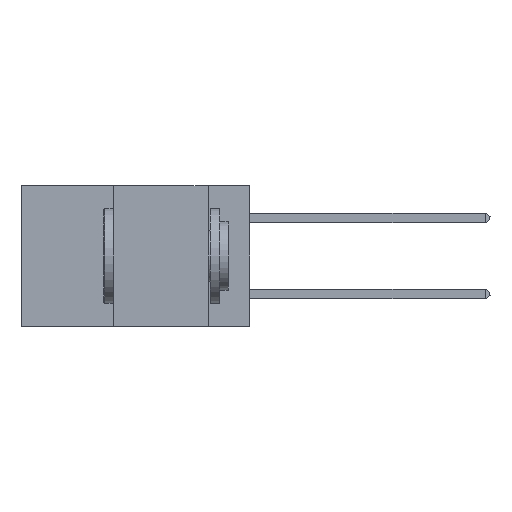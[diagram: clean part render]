
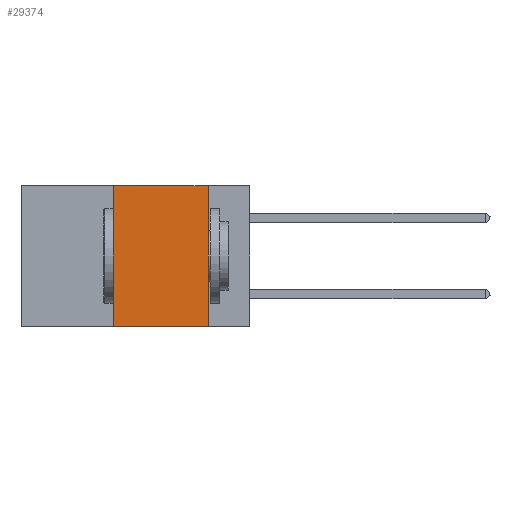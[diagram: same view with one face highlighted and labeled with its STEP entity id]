
A CAD part, left-side view. The second image highlights one B-rep face of the part: STEP entity #29374.
In plain terms, the highlighted planar face has unit normal (-1, 0, 0).
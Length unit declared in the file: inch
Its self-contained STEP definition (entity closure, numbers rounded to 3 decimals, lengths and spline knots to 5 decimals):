
#722 = EDGE_CURVE ( 'NONE', #38622, #37734, #21230, .T. ) ;
#1094 = EDGE_CURVE ( 'NONE', #31111, #38622, #18928, .T. ) ;
#1618 = VECTOR ( 'NONE', #26236, 39.37008 ) ;
#3147 = EDGE_CURVE ( 'NONE', #31111, #35357, #33803, .T. ) ;
#4628 = DIRECTION ( 'NONE',  ( 0., -1., 0. ) ) ;
#5275 = ORIENTED_EDGE ( 'NONE', *, *, #5376, .F. ) ;
#5376 = EDGE_CURVE ( 'NONE', #37734, #35357, #9614, .T. ) ;
#6273 = DIRECTION ( 'NONE',  ( 0., -1., 0. ) ) ;
#9145 = DIRECTION ( 'NONE',  ( 1., 0., 0. ) ) ;
#9614 = LINE ( 'NONE', #11068, #1618 ) ;
#10119 = FACE_OUTER_BOUND ( 'NONE', #15375, .T. ) ;
#10669 = CARTESIAN_POINT ( 'NONE',  ( 0., 0.6, 0. ) ) ;
#11068 = CARTESIAN_POINT ( 'NONE',  ( 0., 0.11, 0. ) ) ;
#11595 = CARTESIAN_POINT ( 'NONE',  ( 0., 0.36, 0. ) ) ;
#11898 = PLANE ( 'NONE',  #23576 ) ;
#13673 = ORIENTED_EDGE ( 'NONE', *, *, #1094, .F. ) ;
#15361 = CARTESIAN_POINT ( 'NONE',  ( 0., 0.36, 0. ) ) ;
#15375 = EDGE_LOOP ( 'NONE', ( #5275, #33425, #13673, #35931 ) ) ;
#15607 = VECTOR ( 'NONE', #27654, 39.37008 ) ;
#18928 = LINE ( 'NONE', #15361, #15607 ) ;
#21230 = LINE ( 'NONE', #10669, #24081 ) ;
#21289 = CARTESIAN_POINT ( 'NONE',  ( 0., 0.6, -0.37 ) ) ;
#23576 = AXIS2_PLACEMENT_3D ( 'NONE', #26832, #9145, #24060 ) ;
#23749 = CARTESIAN_POINT ( 'NONE',  ( 0., 0.11, -0.37 ) ) ;
#24060 = DIRECTION ( 'NONE',  ( 0., 0., -1. ) ) ;
#24081 = VECTOR ( 'NONE', #4628, 39.37008 ) ;
#26236 = DIRECTION ( 'NONE',  ( 0., 0., -1. ) ) ;
#26832 = CARTESIAN_POINT ( 'NONE',  ( 0., 0.6, 0. ) ) ;
#27654 = DIRECTION ( 'NONE',  ( 0., 0., 1. ) ) ;
#29374 = ADVANCED_FACE ( 'NONE', ( #10119 ), #11898, .F. ) ;
#31111 = VERTEX_POINT ( 'NONE', #36740 ) ;
#33425 = ORIENTED_EDGE ( 'NONE', *, *, #722, .F. ) ;
#33803 = LINE ( 'NONE', #21289, #37102 ) ;
#34658 = CARTESIAN_POINT ( 'NONE',  ( 0., 0.11, 0. ) ) ;
#35357 = VERTEX_POINT ( 'NONE', #23749 ) ;
#35931 = ORIENTED_EDGE ( 'NONE', *, *, #3147, .T. ) ;
#36740 = CARTESIAN_POINT ( 'NONE',  ( 0., 0.36, -0.37 ) ) ;
#37102 = VECTOR ( 'NONE', #6273, 39.37008 ) ;
#37734 = VERTEX_POINT ( 'NONE', #34658 ) ;
#38622 = VERTEX_POINT ( 'NONE', #11595 ) ;
